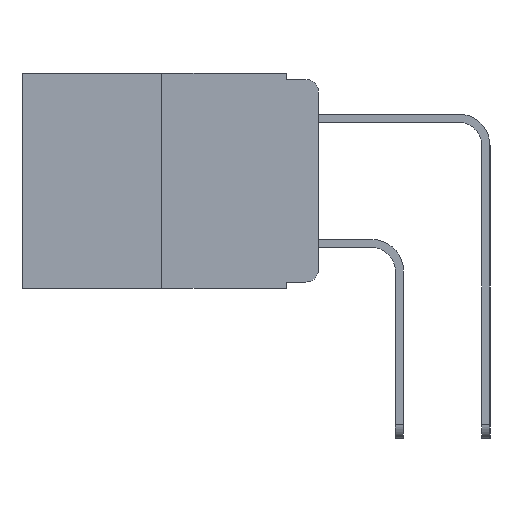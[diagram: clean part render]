
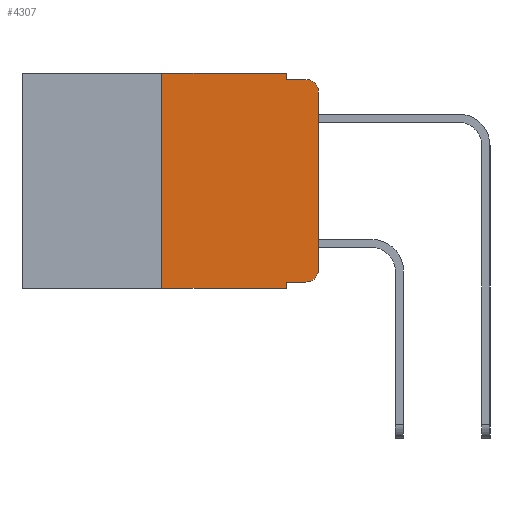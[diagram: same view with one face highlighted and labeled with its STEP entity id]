
A CAD part, left-side view. The second image highlights one B-rep face of the part: STEP entity #4307.
In plain terms, the highlighted planar face has unit normal (-1, 0, 0).
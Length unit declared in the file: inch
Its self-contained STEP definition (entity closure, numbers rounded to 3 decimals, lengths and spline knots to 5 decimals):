
#138 = AXIS2_PLACEMENT_3D ( 'NONE', #6764, #6825, #16014 ) ;
#458 = LINE ( 'NONE', #15852, #13438 ) ;
#573 = ORIENTED_EDGE ( 'NONE', *, *, #5254, .F. ) ;
#1291 = DIRECTION ( 'NONE',  ( 0., 0., -1. ) ) ;
#1500 = VERTEX_POINT ( 'NONE', #13185 ) ;
#1635 = CARTESIAN_POINT ( 'NONE',  ( 0., 0.473, -0.343 ) ) ;
#1817 = DIRECTION ( 'NONE',  ( 1., 0., 0. ) ) ;
#2085 = ORIENTED_EDGE ( 'NONE', *, *, #2772, .T. ) ;
#2364 = DIRECTION ( 'NONE',  ( 0., 0., 1. ) ) ;
#2566 = VERTEX_POINT ( 'NONE', #6708 ) ;
#2719 = CARTESIAN_POINT ( 'NONE',  ( 0., 0.473, 0. ) ) ;
#2772 = EDGE_CURVE ( 'NONE', #12484, #1500, #8647, .T. ) ;
#2824 = LINE ( 'NONE', #2719, #12297 ) ;
#2936 = ORIENTED_EDGE ( 'NONE', *, *, #5634, .F. ) ;
#2943 = DIRECTION ( 'NONE',  ( 0., -1., 0. ) ) ;
#3063 = CARTESIAN_POINT ( 'NONE',  ( 0., 0.473, 0. ) ) ;
#3077 = LINE ( 'NONE', #14884, #9323 ) ;
#3091 = CARTESIAN_POINT ( 'NONE',  ( 0., 0.051, -0.343 ) ) ;
#3215 = VERTEX_POINT ( 'NONE', #13468 ) ;
#3712 = DIRECTION ( 'NONE',  ( 0., 0., -1. ) ) ;
#3951 = ORIENTED_EDGE ( 'NONE', *, *, #12190, .T. ) ;
#3962 = EDGE_CURVE ( 'NONE', #2566, #6252, #5687, .T. ) ;
#3982 = ORIENTED_EDGE ( 'NONE', *, *, #6281, .F. ) ;
#3991 = CARTESIAN_POINT ( 'NONE',  ( 0., 0.25, 0. ) ) ;
#4089 = DIRECTION ( 'NONE',  ( -1., 0., 0. ) ) ;
#4092 = CARTESIAN_POINT ( 'NONE',  ( 0., 0.02, -0.313 ) ) ;
#4307 = ADVANCED_FACE ( 'NONE', ( #6044 ), #6466, .F. ) ;
#4338 = CARTESIAN_POINT ( 'NONE',  ( 0., 0.051, 0. ) ) ;
#4365 = CARTESIAN_POINT ( 'NONE',  ( 0., 0.051, 0. ) ) ;
#4698 = VERTEX_POINT ( 'NONE', #4365 ) ;
#4916 = DIRECTION ( 'NONE',  ( 0., 0., -1. ) ) ;
#5254 = EDGE_CURVE ( 'NONE', #4698, #9251, #14949, .T. ) ;
#5388 = CARTESIAN_POINT ( 'NONE',  ( 0., 0.051, -0.333 ) ) ;
#5539 = VECTOR ( 'NONE', #2943, 39.37008 ) ;
#5554 = VECTOR ( 'NONE', #8455, 39.37008 ) ;
#5628 = LINE ( 'NONE', #3991, #8537 ) ;
#5634 = EDGE_CURVE ( 'NONE', #3215, #16079, #5628, .T. ) ;
#5641 = VECTOR ( 'NONE', #10523, 39.37008 ) ;
#5687 = CIRCLE ( 'NONE', #6181, 0.02 ) ;
#5775 = CARTESIAN_POINT ( 'NONE',  ( 0., 0., -0.03 ) ) ;
#5925 = ORIENTED_EDGE ( 'NONE', *, *, #8860, .F. ) ;
#6044 = FACE_OUTER_BOUND ( 'NONE', #8117, .T. ) ;
#6134 = EDGE_CURVE ( 'NONE', #6252, #12484, #458, .T. ) ;
#6181 = AXIS2_PLACEMENT_3D ( 'NONE', #4092, #4089, #4916 ) ;
#6252 = VERTEX_POINT ( 'NONE', #13719 ) ;
#6281 = EDGE_CURVE ( 'NONE', #16079, #4698, #2824, .T. ) ;
#6284 = LINE ( 'NONE', #1635, #5539 ) ;
#6466 = PLANE ( 'NONE',  #9999 ) ;
#6708 = CARTESIAN_POINT ( 'NONE',  ( 0., 0.02, -0.333 ) ) ;
#6764 = CARTESIAN_POINT ( 'NONE',  ( 0., 0.02, -0.03 ) ) ;
#6825 = DIRECTION ( 'NONE',  ( -1., 0., 0. ) ) ;
#7190 = CARTESIAN_POINT ( 'NONE',  ( 0., 0.051, -0.333 ) ) ;
#7639 = VECTOR ( 'NONE', #3712, 39.37008 ) ;
#7715 = DIRECTION ( 'NONE',  ( 0., -1., 0. ) ) ;
#7850 = EDGE_CURVE ( 'NONE', #3215, #8557, #6284, .T. ) ;
#8033 = ORIENTED_EDGE ( 'NONE', *, *, #10160, .F. ) ;
#8117 = EDGE_LOOP ( 'NONE', ( #12610, #2085, #8033, #573, #3982, #2936, #9950, #5925, #3951, #15958 ) ) ;
#8455 = DIRECTION ( 'NONE',  ( 0., -1., 0. ) ) ;
#8537 = VECTOR ( 'NONE', #10126, 39.37008 ) ;
#8557 = VERTEX_POINT ( 'NONE', #3091 ) ;
#8647 = CIRCLE ( 'NONE', #138, 0.02 ) ;
#8860 = EDGE_CURVE ( 'NONE', #15219, #8557, #12968, .T. ) ;
#9251 = VERTEX_POINT ( 'NONE', #15494 ) ;
#9323 = VECTOR ( 'NONE', #12497, 39.37008 ) ;
#9950 = ORIENTED_EDGE ( 'NONE', *, *, #7850, .T. ) ;
#9999 = AXIS2_PLACEMENT_3D ( 'NONE', #3063, #1817, #1291 ) ;
#10126 = DIRECTION ( 'NONE',  ( 0., 0., 1. ) ) ;
#10160 = EDGE_CURVE ( 'NONE', #9251, #1500, #3077, .T. ) ;
#10523 = DIRECTION ( 'NONE',  ( 0., 0., -1. ) ) ;
#12190 = EDGE_CURVE ( 'NONE', #15219, #2566, #15240, .T. ) ;
#12297 = VECTOR ( 'NONE', #7715, 39.37008 ) ;
#12320 = CARTESIAN_POINT ( 'NONE',  ( 0., 0.051, 0. ) ) ;
#12484 = VERTEX_POINT ( 'NONE', #5775 ) ;
#12497 = DIRECTION ( 'NONE',  ( 0., -1., 0. ) ) ;
#12610 = ORIENTED_EDGE ( 'NONE', *, *, #6134, .T. ) ;
#12968 = LINE ( 'NONE', #12320, #7639 ) ;
#13185 = CARTESIAN_POINT ( 'NONE',  ( 0., 0.02, -0.01 ) ) ;
#13438 = VECTOR ( 'NONE', #2364, 39.37008 ) ;
#13468 = CARTESIAN_POINT ( 'NONE',  ( 0., 0.25, -0.343 ) ) ;
#13719 = CARTESIAN_POINT ( 'NONE',  ( 0., 0., -0.313 ) ) ;
#14884 = CARTESIAN_POINT ( 'NONE',  ( 0., 0.051, -0.01 ) ) ;
#14949 = LINE ( 'NONE', #4338, #5641 ) ;
#15131 = CARTESIAN_POINT ( 'NONE',  ( 0., 0.25, 0. ) ) ;
#15219 = VERTEX_POINT ( 'NONE', #5388 ) ;
#15240 = LINE ( 'NONE', #7190, #5554 ) ;
#15494 = CARTESIAN_POINT ( 'NONE',  ( 0., 0.051, -0.01 ) ) ;
#15852 = CARTESIAN_POINT ( 'NONE',  ( 0., 0., 0. ) ) ;
#15958 = ORIENTED_EDGE ( 'NONE', *, *, #3962, .T. ) ;
#16014 = DIRECTION ( 'NONE',  ( 0., 0., -1. ) ) ;
#16079 = VERTEX_POINT ( 'NONE', #15131 ) ;
